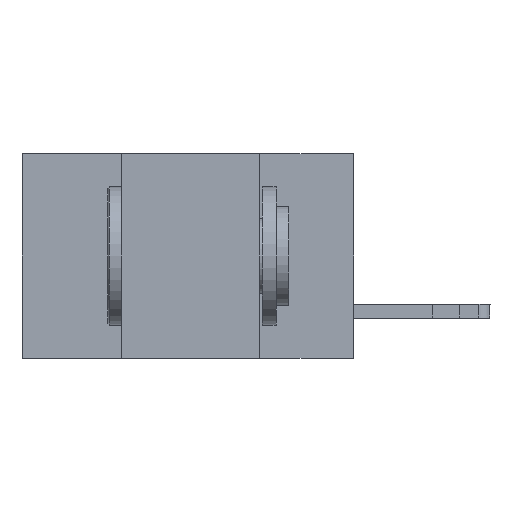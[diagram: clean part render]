
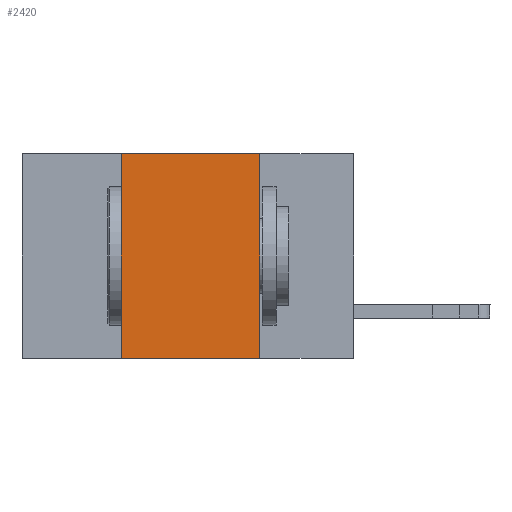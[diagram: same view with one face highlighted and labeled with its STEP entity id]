
A CAD part, left-side view. The second image highlights one B-rep face of the part: STEP entity #2420.
In plain terms, the highlighted planar face has unit normal (-1, 0, 0).
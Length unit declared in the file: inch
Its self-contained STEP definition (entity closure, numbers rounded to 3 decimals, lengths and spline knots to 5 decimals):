
#29 = VERTEX_POINT ( 'NONE', #15530 ) ;
#1012 = CARTESIAN_POINT ( 'NONE',  ( 0., 0.6, 0. ) ) ;
#1924 = VECTOR ( 'NONE', #13000, 39.37008 ) ;
#2171 = ORIENTED_EDGE ( 'NONE', *, *, #9049, .T. ) ;
#2420 = ADVANCED_FACE ( 'NONE', ( #11897 ), #7033, .F. ) ;
#2696 = DIRECTION ( 'NONE',  ( 0., -1., 0. ) ) ;
#2700 = EDGE_CURVE ( 'NONE', #12689, #29, #5099, .T. ) ;
#3307 = EDGE_CURVE ( 'NONE', #4239, #8674, #4579, .T. ) ;
#4239 = VERTEX_POINT ( 'NONE', #8944 ) ;
#4579 = LINE ( 'NONE', #11796, #1924 ) ;
#4772 = EDGE_CURVE ( 'NONE', #29, #4239, #13384, .T. ) ;
#4911 = VECTOR ( 'NONE', #14306, 39.37008 ) ;
#5099 = LINE ( 'NONE', #13083, #4911 ) ;
#5315 = AXIS2_PLACEMENT_3D ( 'NONE', #1012, #12154, #9842 ) ;
#5914 = DIRECTION ( 'NONE',  ( 0., -1., 0. ) ) ;
#6335 = CARTESIAN_POINT ( 'NONE',  ( 0., 0.42, -0.37 ) ) ;
#6600 = VECTOR ( 'NONE', #5914, 39.37008 ) ;
#7033 = PLANE ( 'NONE',  #5315 ) ;
#7370 = VECTOR ( 'NONE', #2696, 39.37008 ) ;
#8674 = VERTEX_POINT ( 'NONE', #12911 ) ;
#8944 = CARTESIAN_POINT ( 'NONE',  ( 0., 0.17, 0. ) ) ;
#9049 = EDGE_CURVE ( 'NONE', #12689, #8674, #15634, .T. ) ;
#9125 = EDGE_LOOP ( 'NONE', ( #14624, #9469, #12338, #2171 ) ) ;
#9469 = ORIENTED_EDGE ( 'NONE', *, *, #4772, .F. ) ;
#9842 = DIRECTION ( 'NONE',  ( 0., 0., -1. ) ) ;
#11796 = CARTESIAN_POINT ( 'NONE',  ( 0., 0.17, 0. ) ) ;
#11897 = FACE_OUTER_BOUND ( 'NONE', #9125, .T. ) ;
#12154 = DIRECTION ( 'NONE',  ( 1., 0., 0. ) ) ;
#12338 = ORIENTED_EDGE ( 'NONE', *, *, #2700, .F. ) ;
#12404 = CARTESIAN_POINT ( 'NONE',  ( 0., 0.6, 0. ) ) ;
#12689 = VERTEX_POINT ( 'NONE', #6335 ) ;
#12911 = CARTESIAN_POINT ( 'NONE',  ( 0., 0.17, -0.37 ) ) ;
#13000 = DIRECTION ( 'NONE',  ( 0., 0., -1. ) ) ;
#13083 = CARTESIAN_POINT ( 'NONE',  ( 0., 0.42, 0. ) ) ;
#13129 = CARTESIAN_POINT ( 'NONE',  ( 0., 0.6, -0.37 ) ) ;
#13384 = LINE ( 'NONE', #12404, #7370 ) ;
#14306 = DIRECTION ( 'NONE',  ( 0., 0., 1. ) ) ;
#14624 = ORIENTED_EDGE ( 'NONE', *, *, #3307, .F. ) ;
#15530 = CARTESIAN_POINT ( 'NONE',  ( 0., 0.42, 0. ) ) ;
#15634 = LINE ( 'NONE', #13129, #6600 ) ;
